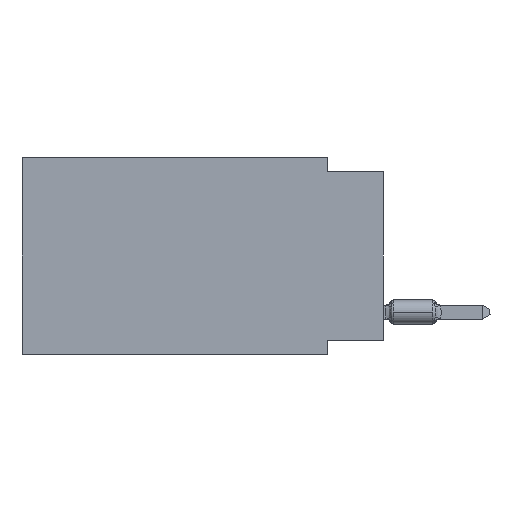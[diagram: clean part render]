
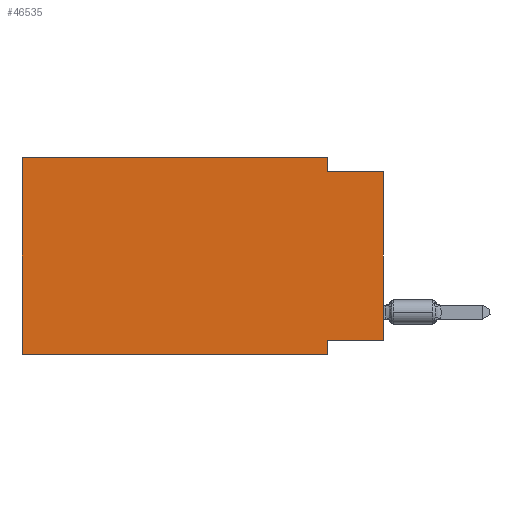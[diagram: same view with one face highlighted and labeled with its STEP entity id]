
A CAD part, left-side view. The second image highlights one B-rep face of the part: STEP entity #46535.
In plain terms, the highlighted planar face has unit normal (-1, 0, 0).
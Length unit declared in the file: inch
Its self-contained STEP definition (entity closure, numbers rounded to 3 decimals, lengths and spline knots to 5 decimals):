
#143 = VERTEX_POINT ( 'NONE', #25796 ) ;
#613 = DIRECTION ( 'NONE',  ( 0., -1., 0. ) ) ;
#751 = VECTOR ( 'NONE', #34033, 39.37008 ) ;
#1223 = CARTESIAN_POINT ( 'NONE',  ( 0., 0.645, 0. ) ) ;
#2364 = ORIENTED_EDGE ( 'NONE', *, *, #37131, .F. ) ;
#2367 = VECTOR ( 'NONE', #42558, 39.37008 ) ;
#3814 = ORIENTED_EDGE ( 'NONE', *, *, #10932, .F. ) ;
#4009 = ORIENTED_EDGE ( 'NONE', *, *, #37059, .T. ) ;
#4029 = CARTESIAN_POINT ( 'NONE',  ( 0., 0., -0.025 ) ) ;
#4664 = CARTESIAN_POINT ( 'NONE',  ( 0., 0.1, 0. ) ) ;
#6612 = ORIENTED_EDGE ( 'NONE', *, *, #49507, .F. ) ;
#7271 = VECTOR ( 'NONE', #613, 39.37008 ) ;
#7946 = CARTESIAN_POINT ( 'NONE',  ( 0., 0.645, 0. ) ) ;
#8540 = CARTESIAN_POINT ( 'NONE',  ( 0., 0.645, 0. ) ) ;
#9083 = LINE ( 'NONE', #8540, #34054 ) ;
#10932 = EDGE_CURVE ( 'NONE', #12263, #19709, #19318, .T. ) ;
#12263 = VERTEX_POINT ( 'NONE', #4664 ) ;
#12544 = DIRECTION ( 'NONE',  ( 0., -1., 0. ) ) ;
#14748 = VECTOR ( 'NONE', #20191, 39.37008 ) ;
#15832 = EDGE_CURVE ( 'NONE', #143, #25237, #46881, .T. ) ;
#16508 = CARTESIAN_POINT ( 'NONE',  ( 0., 0.645, -0.35 ) ) ;
#16727 = CARTESIAN_POINT ( 'NONE',  ( 0., 0., -0.325 ) ) ;
#16782 = VERTEX_POINT ( 'NONE', #52528 ) ;
#16787 = EDGE_LOOP ( 'NONE', ( #4009, #45373, #3814, #29133, #6612, #26262, #2364, #50602 ) ) ;
#18736 = DIRECTION ( 'NONE',  ( 0., 0., -1. ) ) ;
#19116 = VECTOR ( 'NONE', #55231, 39.37008 ) ;
#19318 = LINE ( 'NONE', #23916, #19116 ) ;
#19709 = VERTEX_POINT ( 'NONE', #23900 ) ;
#20191 = DIRECTION ( 'NONE',  ( 0., 0., -1. ) ) ;
#20492 = CARTESIAN_POINT ( 'NONE',  ( 0., 0.1, -0.35 ) ) ;
#20723 = VERTEX_POINT ( 'NONE', #50939 ) ;
#22764 = FACE_OUTER_BOUND ( 'NONE', #16787, .T. ) ;
#23900 = CARTESIAN_POINT ( 'NONE',  ( 0., 0.1, -0.025 ) ) ;
#23916 = CARTESIAN_POINT ( 'NONE',  ( 0., 0.1, 0. ) ) ;
#25237 = VERTEX_POINT ( 'NONE', #28771 ) ;
#25452 = DIRECTION ( 'NONE',  ( 0., 0., 1. ) ) ;
#25796 = CARTESIAN_POINT ( 'NONE',  ( 0., 0., -0.325 ) ) ;
#26262 = ORIENTED_EDGE ( 'NONE', *, *, #40683, .T. ) ;
#27959 = DIRECTION ( 'NONE',  ( 0., 0., 1. ) ) ;
#28771 = CARTESIAN_POINT ( 'NONE',  ( 0., 0.1, -0.325 ) ) ;
#29133 = ORIENTED_EDGE ( 'NONE', *, *, #39263, .F. ) ;
#29388 = VECTOR ( 'NONE', #27959, 39.37008 ) ;
#30303 = VECTOR ( 'NONE', #25452, 39.37008 ) ;
#31619 = CARTESIAN_POINT ( 'NONE',  ( 0., 0.645, 0. ) ) ;
#32547 = CARTESIAN_POINT ( 'NONE',  ( 0., 0., 0. ) ) ;
#33160 = AXIS2_PLACEMENT_3D ( 'NONE', #1223, #40271, #18736 ) ;
#33689 = LINE ( 'NONE', #20492, #14748 ) ;
#34033 = DIRECTION ( 'NONE',  ( 0., -1., 0. ) ) ;
#34054 = VECTOR ( 'NONE', #12544, 39.37008 ) ;
#35373 = LINE ( 'NONE', #43429, #7271 ) ;
#37059 = EDGE_CURVE ( 'NONE', #143, #42117, #54662, .T. ) ;
#37131 = EDGE_CURVE ( 'NONE', #25237, #20723, #33689, .T. ) ;
#38048 = LINE ( 'NONE', #16508, #751 ) ;
#39263 = EDGE_CURVE ( 'NONE', #43021, #12263, #9083, .T. ) ;
#39740 = PLANE ( 'NONE',  #33160 ) ;
#40271 = DIRECTION ( 'NONE',  ( 1., 0., 0. ) ) ;
#40683 = EDGE_CURVE ( 'NONE', #16782, #20723, #38048, .T. ) ;
#41627 = EDGE_CURVE ( 'NONE', #19709, #42117, #35373, .T. ) ;
#42117 = VERTEX_POINT ( 'NONE', #4029 ) ;
#42558 = DIRECTION ( 'NONE',  ( 0., 1., 0. ) ) ;
#43021 = VERTEX_POINT ( 'NONE', #31619 ) ;
#43429 = CARTESIAN_POINT ( 'NONE',  ( 0., 0., -0.025 ) ) ;
#45373 = ORIENTED_EDGE ( 'NONE', *, *, #41627, .F. ) ;
#46535 = ADVANCED_FACE ( 'NONE', ( #22764 ), #39740, .F. ) ;
#46881 = LINE ( 'NONE', #16727, #2367 ) ;
#47017 = LINE ( 'NONE', #7946, #30303 ) ;
#49507 = EDGE_CURVE ( 'NONE', #16782, #43021, #47017, .T. ) ;
#50602 = ORIENTED_EDGE ( 'NONE', *, *, #15832, .F. ) ;
#50939 = CARTESIAN_POINT ( 'NONE',  ( 0., 0.1, -0.35 ) ) ;
#52528 = CARTESIAN_POINT ( 'NONE',  ( 0., 0.645, -0.35 ) ) ;
#54662 = LINE ( 'NONE', #32547, #29388 ) ;
#55231 = DIRECTION ( 'NONE',  ( 0., 0., -1. ) ) ;
